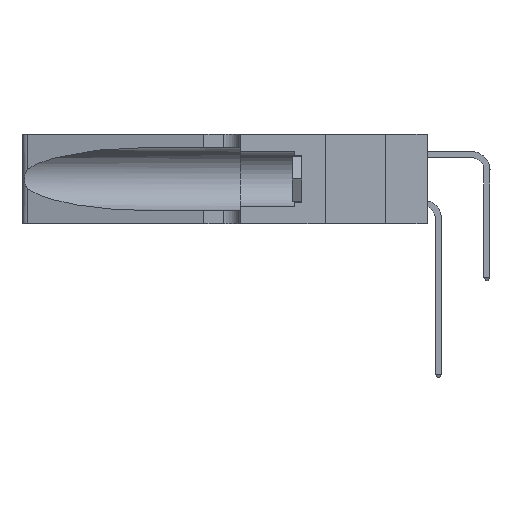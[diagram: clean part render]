
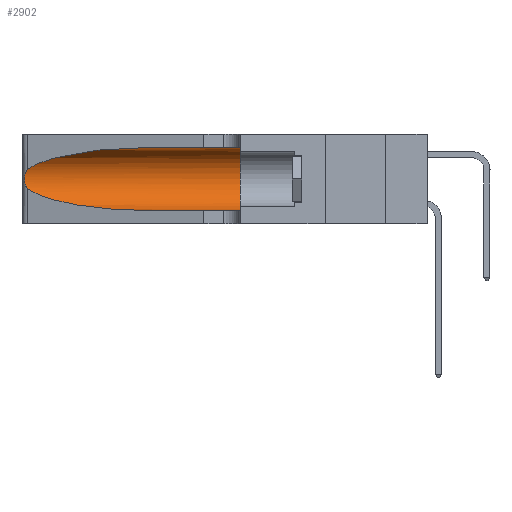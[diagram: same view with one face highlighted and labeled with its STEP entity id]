
A CAD part, left-side view. The second image highlights one B-rep face of the part: STEP entity #2902.
In plain terms, the highlighted cylindrical face has radius 3.308 mm (diameter 6.617 mm), a partial arc.
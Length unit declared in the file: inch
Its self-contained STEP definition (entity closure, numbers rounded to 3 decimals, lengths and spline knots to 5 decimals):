
#473 = DIRECTION ( 'NONE',  ( 0., -1., 0. ) ) ;
#1419 = EDGE_CURVE ( 'NONE', #4776, #4996, #9190, .T. ) ;
#2902 = ADVANCED_FACE ( 'NONE', ( #5425 ), #10490, .F. ) ;
#3090 = CARTESIAN_POINT ( 'NONE',  ( 0.26075, 1.23896, 0.178 ) ) ;
#4099 = AXIS2_PLACEMENT_3D ( 'NONE', #5737, #18577, #8620 ) ;
#4610 = ORIENTED_EDGE ( 'NONE', *, *, #1419, .F. ) ;
#4776 = VERTEX_POINT ( 'NONE', #8498 ) ;
#4996 = VERTEX_POINT ( 'NONE', #5171 ) ;
#5151 = CARTESIAN_POINT ( 'NONE',  ( 0.25555, 1.22994, 0.2215 ) ) ;
#5171 = CARTESIAN_POINT ( 'NONE',  ( 0.1305, 0.35, 0.31525 ) ) ;
#5425 = FACE_OUTER_BOUND ( 'NONE', #21942, .T. ) ;
#5737 = CARTESIAN_POINT ( 'NONE',  ( 0.1305, 0.35, 0.185 ) ) ;
#5967 = CARTESIAN_POINT ( 'NONE',  ( 0.25487, 1.22718, 0.14631 ) ) ;
#7128 = CARTESIAN_POINT ( 'NONE',  ( 0.25789, 1.23486, 0.15765 ) ) ;
#7228 =( BOUNDED_CURVE ( )  B_SPLINE_CURVE ( 3, ( #5967, #20803, #22993, #9921 ),
 .UNSPECIFIED., .F., .F. ) 
 B_SPLINE_CURVE_WITH_KNOTS ( ( 4, 4 ),
 ( 3.44316, 4.71239 ),
 .UNSPECIFIED. ) 
 CURVE ( )  GEOMETRIC_REPRESENTATION_ITEM ( )  RATIONAL_B_SPLINE_CURVE ( ( 1., 0.87, 0.87, 1. ) ) 
 REPRESENTATION_ITEM ( '' )  );
#7311 = CARTESIAN_POINT ( 'NONE',  ( 0.25639, 1.23184, 0.21858 ) ) ;
#7984 = CARTESIAN_POINT ( 'NONE',  ( 0.25487, 1.22718, 0.14631 ) ) ;
#8099 = CARTESIAN_POINT ( 'NONE',  ( 0.1305, 0.72297, 0.05475 ) ) ;
#8498 = CARTESIAN_POINT ( 'NONE',  ( 0.1305, 0.72297, 0.31525 ) ) ;
#8620 = DIRECTION ( 'NONE',  ( 0., 0., 1. ) ) ;
#8962 = EDGE_CURVE ( 'NONE', #26376, #19270, #21008, .T. ) ;
#9190 = LINE ( 'NONE', #12563, #9864 ) ;
#9430 = ORIENTED_EDGE ( 'NONE', *, *, #17412, .F. ) ;
#9473 = CARTESIAN_POINT ( 'NONE',  ( 0.26075, 1.23896, 0.19203 ) ) ;
#9578 = VERTEX_POINT ( 'NONE', #13412 ) ;
#9864 = VECTOR ( 'NONE', #21272, 39.37008 ) ;
#9921 = CARTESIAN_POINT ( 'NONE',  ( 0.1305, 0.72297, 0.05475 ) ) ;
#10490 = CYLINDRICAL_SURFACE ( 'NONE', #27791, 0.13025 ) ;
#11031 =( BOUNDED_CURVE ( )  B_SPLINE_CURVE ( 3, ( #25942, #16091, #24946, #12316 ),
 .UNSPECIFIED., .F., .F. ) 
 B_SPLINE_CURVE_WITH_KNOTS ( ( 4, 4 ),
 ( 1.5708, 2.84003 ),
 .UNSPECIFIED. ) 
 CURVE ( )  GEOMETRIC_REPRESENTATION_ITEM ( )  RATIONAL_B_SPLINE_CURVE ( ( 1., 0.87, 0.87, 1. ) ) 
 REPRESENTATION_ITEM ( '' )  );
#12302 = VECTOR ( 'NONE', #473, 39.37008 ) ;
#12316 = CARTESIAN_POINT ( 'NONE',  ( 0.25487, 1.22718, 0.22369 ) ) ;
#12563 = CARTESIAN_POINT ( 'NONE',  ( 0.1305, 1.61858, 0.31525 ) ) ;
#12953 = ORIENTED_EDGE ( 'NONE', *, *, #25198, .T. ) ;
#13212 = DIRECTION ( 'NONE',  ( 0., -1., 0. ) ) ;
#13412 = CARTESIAN_POINT ( 'NONE',  ( 0.1305, 0.35, 0.05475 ) ) ;
#13419 = CARTESIAN_POINT ( 'NONE',  ( 0.25487, 1.22718, 0.14631 ) ) ;
#15958 = CARTESIAN_POINT ( 'NONE',  ( 0.25856, 1.23593, 0.16098 ) ) ;
#16091 = CARTESIAN_POINT ( 'NONE',  ( 0.18966, 0.96281, 0.31525 ) ) ;
#17412 = EDGE_CURVE ( 'NONE', #4996, #9578, #19150, .T. ) ;
#17429 = CARTESIAN_POINT ( 'NONE',  ( 0.1305, 1.61858, 0.185 ) ) ;
#18000 = CARTESIAN_POINT ( 'NONE',  ( 0.25487, 1.22718, 0.22369 ) ) ;
#18078 = DIRECTION ( 'NONE',  ( 0., 0., -1. ) ) ;
#18577 = DIRECTION ( 'NONE',  ( 0., 1., 0. ) ) ;
#19150 = CIRCLE ( 'NONE', #4099, 0.13025 ) ;
#19270 = VERTEX_POINT ( 'NONE', #7984 ) ;
#19585 = EDGE_CURVE ( 'NONE', #20137, #9578, #26040, .T. ) ;
#19750 = CARTESIAN_POINT ( 'NONE',  ( 0.1305, 1.61858, 0.05475 ) ) ;
#19982 = CARTESIAN_POINT ( 'NONE',  ( 0.25787, 1.23484, 0.2124 ) ) ;
#20137 = VERTEX_POINT ( 'NONE', #8099 ) ;
#20803 = CARTESIAN_POINT ( 'NONE',  ( 0.2373, 1.15595, 0.08982 ) ) ;
#21008 = B_SPLINE_CURVE_WITH_KNOTS ( 'NONE', 3,
 ( #18000, #5151, #7311, #19982, #22359, #22455, #9473, #3090, #24510, #15958, #7128, #24601, #26279, #13419 ),
 .UNSPECIFIED., .F., .F.,
 ( 4, 2, 2, 2, 2, 2, 4 ),
 ( 0., 0.00027, 0.00053, 0.00107, 0.0016, 0.00187, 0.00214 ),
 .UNSPECIFIED. ) ;
#21272 = DIRECTION ( 'NONE',  ( 0., -1., 0. ) ) ;
#21942 = EDGE_LOOP ( 'NONE', ( #22514, #26648, #12953, #23589, #9430, #4610 ) ) ;
#22359 = CARTESIAN_POINT ( 'NONE',  ( 0.25854, 1.2359, 0.20912 ) ) ;
#22455 = CARTESIAN_POINT ( 'NONE',  ( 0.26018, 1.23835, 0.19895 ) ) ;
#22514 = ORIENTED_EDGE ( 'NONE', *, *, #25918, .T. ) ;
#22993 = CARTESIAN_POINT ( 'NONE',  ( 0.18966, 0.96281, 0.05475 ) ) ;
#23589 = ORIENTED_EDGE ( 'NONE', *, *, #19585, .T. ) ;
#24510 = CARTESIAN_POINT ( 'NONE',  ( 0.26017, 1.23833, 0.17102 ) ) ;
#24601 = CARTESIAN_POINT ( 'NONE',  ( 0.25639, 1.23186, 0.15144 ) ) ;
#24923 = CARTESIAN_POINT ( 'NONE',  ( 0.25487, 1.22718, 0.22369 ) ) ;
#24946 = CARTESIAN_POINT ( 'NONE',  ( 0.2373, 1.15595, 0.28018 ) ) ;
#25198 = EDGE_CURVE ( 'NONE', #19270, #20137, #7228, .T. ) ;
#25918 = EDGE_CURVE ( 'NONE', #4776, #26376, #11031, .T. ) ;
#25942 = CARTESIAN_POINT ( 'NONE',  ( 0.1305, 0.72297, 0.31525 ) ) ;
#26040 = LINE ( 'NONE', #19750, #12302 ) ;
#26279 = CARTESIAN_POINT ( 'NONE',  ( 0.25555, 1.22993, 0.14849 ) ) ;
#26376 = VERTEX_POINT ( 'NONE', #24923 ) ;
#26648 = ORIENTED_EDGE ( 'NONE', *, *, #8962, .T. ) ;
#27791 = AXIS2_PLACEMENT_3D ( 'NONE', #17429, #13212, #18078 ) ;
